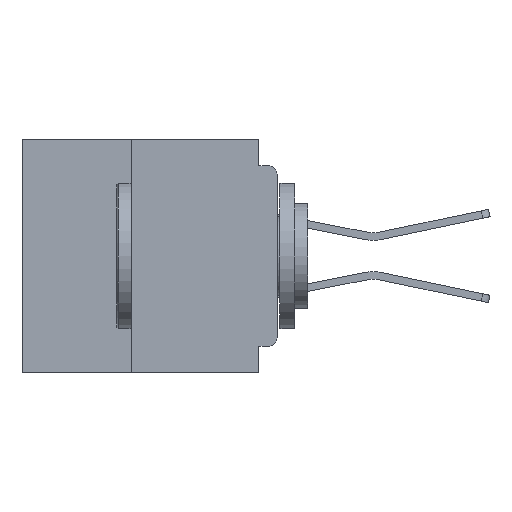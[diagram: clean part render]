
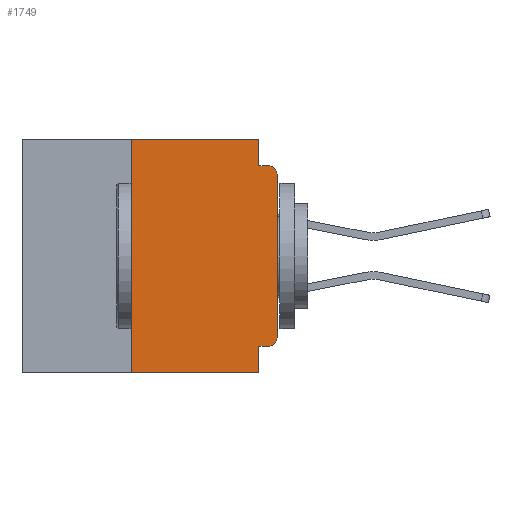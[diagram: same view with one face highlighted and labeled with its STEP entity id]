
A CAD part, left-side view. The second image highlights one B-rep face of the part: STEP entity #1749.
In plain terms, the highlighted planar face has unit normal (-1, 0, 0).
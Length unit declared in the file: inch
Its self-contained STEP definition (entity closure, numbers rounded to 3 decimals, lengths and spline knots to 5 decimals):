
#939 = VERTEX_POINT ( 'NONE', #17764 ) ;
#1044 = EDGE_CURVE ( 'NONE', #939, #16343, #19916, .T. ) ;
#1749 = ADVANCED_FACE ( 'NONE', ( #7547 ), #41353, .F. ) ;
#2313 = EDGE_CURVE ( 'NONE', #36314, #10521, #42864, .T. ) ;
#5515 = VECTOR ( 'NONE', #31030, 39.37008 ) ;
#6808 = VECTOR ( 'NONE', #34391, 39.37008 ) ;
#6998 = ORIENTED_EDGE ( 'NONE', *, *, #1044, .T. ) ;
#7547 = FACE_OUTER_BOUND ( 'NONE', #42068, .T. ) ;
#9417 = EDGE_CURVE ( 'NONE', #10521, #16343, #38799, .T. ) ;
#10521 = VERTEX_POINT ( 'NONE', #50190 ) ;
#10950 = DIRECTION ( 'NONE',  ( 0., -1., 0. ) ) ;
#11107 = DIRECTION ( 'NONE',  ( 0., 0., -1. ) ) ;
#11226 = CARTESIAN_POINT ( 'NONE',  ( 0., 0.015, -0.06 ) ) ;
#11238 = DIRECTION ( 'NONE',  ( -1., 0., 0. ) ) ;
#11830 = ORIENTED_EDGE ( 'NONE', *, *, #23823, .T. ) ;
#11865 = CARTESIAN_POINT ( 'NONE',  ( 0., 0., -0.34 ) ) ;
#14362 = VERTEX_POINT ( 'NONE', #19545 ) ;
#15028 = VERTEX_POINT ( 'NONE', #31097 ) ;
#15086 = ORIENTED_EDGE ( 'NONE', *, *, #18859, .T. ) ;
#15613 = EDGE_CURVE ( 'NONE', #25527, #14362, #17110, .T. ) ;
#15881 = DIRECTION ( 'NONE',  ( 0., -1., 0. ) ) ;
#16343 = VERTEX_POINT ( 'NONE', #31327 ) ;
#16980 = LINE ( 'NONE', #22274, #51655 ) ;
#17110 = LINE ( 'NONE', #39573, #5515 ) ;
#17764 = CARTESIAN_POINT ( 'NONE',  ( 0., 0., -0.06 ) ) ;
#17907 = CARTESIAN_POINT ( 'NONE',  ( 0., 0.031, -0.355 ) ) ;
#18094 = CARTESIAN_POINT ( 'NONE',  ( 0., 0., -0.355 ) ) ;
#18401 = LINE ( 'NONE', #30032, #6808 ) ;
#18859 = EDGE_CURVE ( 'NONE', #15028, #45424, #33825, .T. ) ;
#19545 = CARTESIAN_POINT ( 'NONE',  ( 0., 0.25, 0. ) ) ;
#19718 = LINE ( 'NONE', #46058, #52995 ) ;
#19916 = CIRCLE ( 'NONE', #33437, 0.015 ) ;
#21726 = CARTESIAN_POINT ( 'NONE',  ( 0., 0.25, -0.4 ) ) ;
#22274 = CARTESIAN_POINT ( 'NONE',  ( 0., 0.437, -0.4 ) ) ;
#22421 = LINE ( 'NONE', #46274, #55624 ) ;
#22511 = DIRECTION ( 'NONE',  ( 0., 1., 0. ) ) ;
#22871 = CARTESIAN_POINT ( 'NONE',  ( 0., 0.031, -0.4 ) ) ;
#23789 = CARTESIAN_POINT ( 'NONE',  ( 0., 0.031, 0. ) ) ;
#23823 = EDGE_CURVE ( 'NONE', #25527, #28655, #16980, .T. ) ;
#24300 = DIRECTION ( 'NONE',  ( -1., 0., 0. ) ) ;
#25527 = VERTEX_POINT ( 'NONE', #21726 ) ;
#26594 = DIRECTION ( 'NONE',  ( 0., 0., -1. ) ) ;
#26776 = CARTESIAN_POINT ( 'NONE',  ( 0., 0.031, 0. ) ) ;
#26805 = EDGE_CURVE ( 'NONE', #15028, #54223, #38673, .T. ) ;
#28655 = VERTEX_POINT ( 'NONE', #22871 ) ;
#29263 = ORIENTED_EDGE ( 'NONE', *, *, #38922, .T. ) ;
#29966 = VECTOR ( 'NONE', #10950, 39.37008 ) ;
#30032 = CARTESIAN_POINT ( 'NONE',  ( 0., 0.031, -0.4 ) ) ;
#30582 = ORIENTED_EDGE ( 'NONE', *, *, #9417, .F. ) ;
#31030 = DIRECTION ( 'NONE',  ( 0., 0., 1. ) ) ;
#31097 = CARTESIAN_POINT ( 'NONE',  ( 0., 0.015, -0.355 ) ) ;
#31327 = CARTESIAN_POINT ( 'NONE',  ( 0., 0.015, -0.045 ) ) ;
#32427 = ORIENTED_EDGE ( 'NONE', *, *, #45833, .F. ) ;
#33437 = AXIS2_PLACEMENT_3D ( 'NONE', #11226, #11238, #11107 ) ;
#33825 = CIRCLE ( 'NONE', #42714, 0.015 ) ;
#34391 = DIRECTION ( 'NONE',  ( 0., 0., -1. ) ) ;
#35871 = ORIENTED_EDGE ( 'NONE', *, *, #15613, .F. ) ;
#36314 = VERTEX_POINT ( 'NONE', #23789 ) ;
#38673 = LINE ( 'NONE', #18094, #48831 ) ;
#38799 = LINE ( 'NONE', #41388, #29966 ) ;
#38922 = EDGE_CURVE ( 'NONE', #45424, #939, #19718, .T. ) ;
#38929 = AXIS2_PLACEMENT_3D ( 'NONE', #41599, #41044, #40983 ) ;
#39573 = CARTESIAN_POINT ( 'NONE',  ( 0., 0.25, -0.4 ) ) ;
#40983 = DIRECTION ( 'NONE',  ( 0., 0., -1. ) ) ;
#41044 = DIRECTION ( 'NONE',  ( 1., 0., 0. ) ) ;
#41353 = PLANE ( 'NONE',  #38929 ) ;
#41388 = CARTESIAN_POINT ( 'NONE',  ( 0., 0., -0.045 ) ) ;
#41599 = CARTESIAN_POINT ( 'NONE',  ( 0., 0.437, 0. ) ) ;
#41683 = DIRECTION ( 'NONE',  ( 0., 0., 1. ) ) ;
#42068 = EDGE_LOOP ( 'NONE', ( #29263, #6998, #30582, #44659, #32427, #35871, #11830, #53111, #56115, #15086 ) ) ;
#42714 = AXIS2_PLACEMENT_3D ( 'NONE', #50299, #24300, #54615 ) ;
#42864 = LINE ( 'NONE', #26776, #44231 ) ;
#44231 = VECTOR ( 'NONE', #26594, 39.37008 ) ;
#44659 = ORIENTED_EDGE ( 'NONE', *, *, #2313, .F. ) ;
#45424 = VERTEX_POINT ( 'NONE', #11865 ) ;
#45833 = EDGE_CURVE ( 'NONE', #14362, #36314, #22421, .T. ) ;
#46058 = CARTESIAN_POINT ( 'NONE',  ( 0., 0., 0. ) ) ;
#46274 = CARTESIAN_POINT ( 'NONE',  ( 0., 0.437, 0. ) ) ;
#48831 = VECTOR ( 'NONE', #22511, 39.37008 ) ;
#50190 = CARTESIAN_POINT ( 'NONE',  ( 0., 0.031, -0.045 ) ) ;
#50299 = CARTESIAN_POINT ( 'NONE',  ( 0., 0.015, -0.34 ) ) ;
#51655 = VECTOR ( 'NONE', #52604, 39.37008 ) ;
#52604 = DIRECTION ( 'NONE',  ( 0., -1., 0. ) ) ;
#52995 = VECTOR ( 'NONE', #41683, 39.37008 ) ;
#53111 = ORIENTED_EDGE ( 'NONE', *, *, #56149, .F. ) ;
#54223 = VERTEX_POINT ( 'NONE', #17907 ) ;
#54615 = DIRECTION ( 'NONE',  ( 0., 0., -1. ) ) ;
#55624 = VECTOR ( 'NONE', #15881, 39.37008 ) ;
#56115 = ORIENTED_EDGE ( 'NONE', *, *, #26805, .F. ) ;
#56149 = EDGE_CURVE ( 'NONE', #54223, #28655, #18401, .T. ) ;
